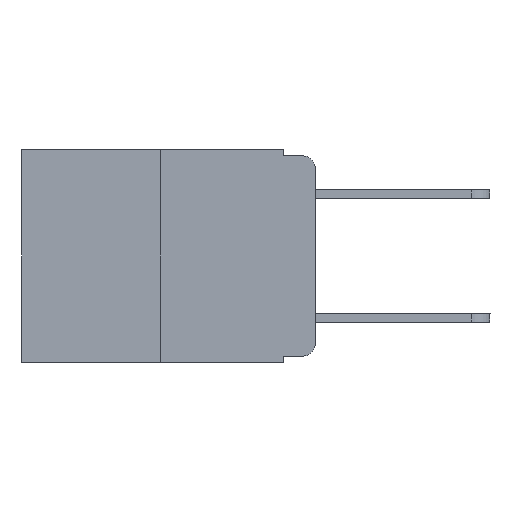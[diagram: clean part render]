
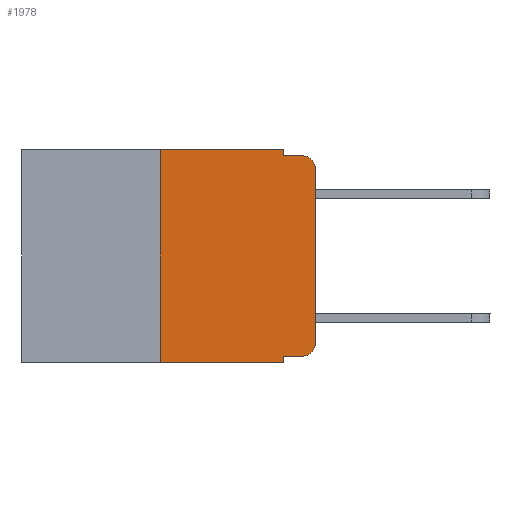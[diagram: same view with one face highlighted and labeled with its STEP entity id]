
A CAD part, left-side view. The second image highlights one B-rep face of the part: STEP entity #1978.
In plain terms, the highlighted planar face has unit normal (-1, 0, 0).
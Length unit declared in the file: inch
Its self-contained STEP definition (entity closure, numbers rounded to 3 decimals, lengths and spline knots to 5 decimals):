
#204 = ORIENTED_EDGE ( 'NONE', *, *, #4005, .F. ) ;
#220 = ORIENTED_EDGE ( 'NONE', *, *, #2629, .F. ) ;
#281 = DIRECTION ( 'NONE',  ( -1., 0., 0. ) ) ;
#466 = DIRECTION ( 'NONE',  ( 0., -1., 0. ) ) ;
#698 = CARTESIAN_POINT ( 'NONE',  ( 0., 0.473, 0. ) ) ;
#937 = CARTESIAN_POINT ( 'NONE',  ( 0., 0.02, -0.03 ) ) ;
#952 = EDGE_CURVE ( 'NONE', #2638, #2480, #9303, .T. ) ;
#1048 = VECTOR ( 'NONE', #466, 39.37008 ) ;
#1066 = PLANE ( 'NONE',  #6768 ) ;
#1190 = CARTESIAN_POINT ( 'NONE',  ( 0., 0., -0.03 ) ) ;
#1874 = CARTESIAN_POINT ( 'NONE',  ( 0., 0.25, 0. ) ) ;
#1978 = ADVANCED_FACE ( 'NONE', ( #4503 ), #1066, .F. ) ;
#2025 = VERTEX_POINT ( 'NONE', #2828 ) ;
#2397 = VECTOR ( 'NONE', #9776, 39.37008 ) ;
#2480 = VERTEX_POINT ( 'NONE', #6492 ) ;
#2524 = LINE ( 'NONE', #11760, #11981 ) ;
#2528 = CARTESIAN_POINT ( 'NONE',  ( 0., 0.051, 0. ) ) ;
#2629 = EDGE_CURVE ( 'NONE', #3227, #7177, #2720, .T. ) ;
#2638 = VERTEX_POINT ( 'NONE', #1190 ) ;
#2720 = LINE ( 'NONE', #3881, #2882 ) ;
#2815 = DIRECTION ( 'NONE',  ( 0., 0., -1. ) ) ;
#2828 = CARTESIAN_POINT ( 'NONE',  ( 0., 0.25, -0.343 ) ) ;
#2833 = EDGE_CURVE ( 'NONE', #3227, #3656, #4493, .T. ) ;
#2882 = VECTOR ( 'NONE', #4822, 39.37008 ) ;
#3107 = ORIENTED_EDGE ( 'NONE', *, *, #6927, .T. ) ;
#3157 = VECTOR ( 'NONE', #9099, 39.37008 ) ;
#3201 = VECTOR ( 'NONE', #8746, 39.37008 ) ;
#3227 = VERTEX_POINT ( 'NONE', #8756 ) ;
#3245 = LINE ( 'NONE', #4155, #1048 ) ;
#3328 = ORIENTED_EDGE ( 'NONE', *, *, #2833, .T. ) ;
#3377 = ORIENTED_EDGE ( 'NONE', *, *, #9603, .T. ) ;
#3656 = VERTEX_POINT ( 'NONE', #9373 ) ;
#3744 = CARTESIAN_POINT ( 'NONE',  ( 0., 0.051, -0.333 ) ) ;
#3881 = CARTESIAN_POINT ( 'NONE',  ( 0., 0.051, 0. ) ) ;
#4005 = EDGE_CURVE ( 'NONE', #2025, #8169, #6362, .T. ) ;
#4155 = CARTESIAN_POINT ( 'NONE',  ( 0., 0.051, -0.01 ) ) ;
#4394 = DIRECTION ( 'NONE',  ( 0., 0., 1. ) ) ;
#4493 = LINE ( 'NONE', #3744, #10304 ) ;
#4503 = FACE_OUTER_BOUND ( 'NONE', #7170, .T. ) ;
#4807 = DIRECTION ( 'NONE',  ( 0., 0., -1. ) ) ;
#4822 = DIRECTION ( 'NONE',  ( 0., 0., -1. ) ) ;
#5575 = EDGE_CURVE ( 'NONE', #8169, #6248, #6537, .T. ) ;
#5698 = DIRECTION ( 'NONE',  ( -1., 0., 0. ) ) ;
#5834 = AXIS2_PLACEMENT_3D ( 'NONE', #937, #5698, #2815 ) ;
#5907 = CARTESIAN_POINT ( 'NONE',  ( 0., 0.02, -0.313 ) ) ;
#6030 = EDGE_CURVE ( 'NONE', #6248, #7051, #6942, .T. ) ;
#6152 = ORIENTED_EDGE ( 'NONE', *, *, #7881, .F. ) ;
#6248 = VERTEX_POINT ( 'NONE', #9352 ) ;
#6362 = LINE ( 'NONE', #7903, #2397 ) ;
#6492 = CARTESIAN_POINT ( 'NONE',  ( 0., 0.02, -0.01 ) ) ;
#6537 = LINE ( 'NONE', #698, #3157 ) ;
#6565 = DIRECTION ( 'NONE',  ( 0., -1., 0. ) ) ;
#6636 = CARTESIAN_POINT ( 'NONE',  ( 0., 0.051, -0.01 ) ) ;
#6768 = AXIS2_PLACEMENT_3D ( 'NONE', #9439, #12054, #4807 ) ;
#6927 = EDGE_CURVE ( 'NONE', #9990, #2638, #2524, .T. ) ;
#6942 = LINE ( 'NONE', #2528, #10418 ) ;
#6987 = CARTESIAN_POINT ( 'NONE',  ( 0., 0.051, -0.343 ) ) ;
#7051 = VERTEX_POINT ( 'NONE', #6636 ) ;
#7170 = EDGE_LOOP ( 'NONE', ( #3107, #11338, #6152, #10719, #9768, #204, #3377, #220, #3328, #11371 ) ) ;
#7177 = VERTEX_POINT ( 'NONE', #6987 ) ;
#7207 = DIRECTION ( 'NONE',  ( 0., 0., -1. ) ) ;
#7565 = CIRCLE ( 'NONE', #10536, 0.02 ) ;
#7881 = EDGE_CURVE ( 'NONE', #7051, #2480, #3245, .T. ) ;
#7903 = CARTESIAN_POINT ( 'NONE',  ( 0., 0.25, 0. ) ) ;
#8169 = VERTEX_POINT ( 'NONE', #1874 ) ;
#8746 = DIRECTION ( 'NONE',  ( 0., -1., 0. ) ) ;
#8756 = CARTESIAN_POINT ( 'NONE',  ( 0., 0.051, -0.333 ) ) ;
#9099 = DIRECTION ( 'NONE',  ( 0., -1., 0. ) ) ;
#9303 = CIRCLE ( 'NONE', #5834, 0.02 ) ;
#9352 = CARTESIAN_POINT ( 'NONE',  ( 0., 0.051, 0. ) ) ;
#9373 = CARTESIAN_POINT ( 'NONE',  ( 0., 0.02, -0.333 ) ) ;
#9431 = LINE ( 'NONE', #9865, #3201 ) ;
#9439 = CARTESIAN_POINT ( 'NONE',  ( 0., 0.473, 0. ) ) ;
#9518 = EDGE_CURVE ( 'NONE', #3656, #9990, #7565, .T. ) ;
#9603 = EDGE_CURVE ( 'NONE', #2025, #7177, #9431, .T. ) ;
#9768 = ORIENTED_EDGE ( 'NONE', *, *, #5575, .F. ) ;
#9776 = DIRECTION ( 'NONE',  ( 0., 0., 1. ) ) ;
#9865 = CARTESIAN_POINT ( 'NONE',  ( 0., 0.473, -0.343 ) ) ;
#9990 = VERTEX_POINT ( 'NONE', #10468 ) ;
#10304 = VECTOR ( 'NONE', #6565, 39.37008 ) ;
#10418 = VECTOR ( 'NONE', #7207, 39.37008 ) ;
#10468 = CARTESIAN_POINT ( 'NONE',  ( 0., 0., -0.313 ) ) ;
#10479 = DIRECTION ( 'NONE',  ( 0., 0., -1. ) ) ;
#10536 = AXIS2_PLACEMENT_3D ( 'NONE', #5907, #281, #10479 ) ;
#10719 = ORIENTED_EDGE ( 'NONE', *, *, #6030, .F. ) ;
#11338 = ORIENTED_EDGE ( 'NONE', *, *, #952, .T. ) ;
#11371 = ORIENTED_EDGE ( 'NONE', *, *, #9518, .T. ) ;
#11760 = CARTESIAN_POINT ( 'NONE',  ( 0., 0., 0. ) ) ;
#11981 = VECTOR ( 'NONE', #4394, 39.37008 ) ;
#12054 = DIRECTION ( 'NONE',  ( 1., 0., 0. ) ) ;
